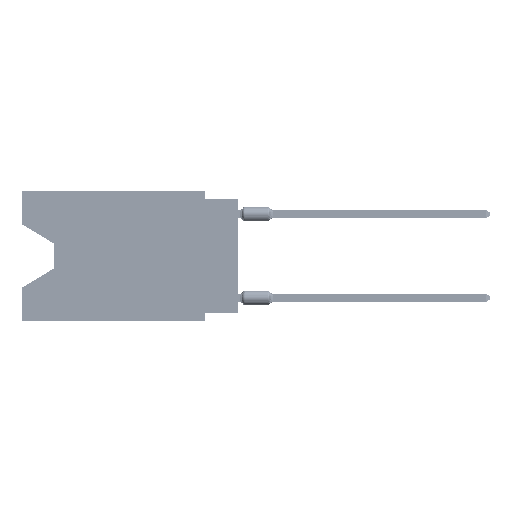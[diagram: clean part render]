
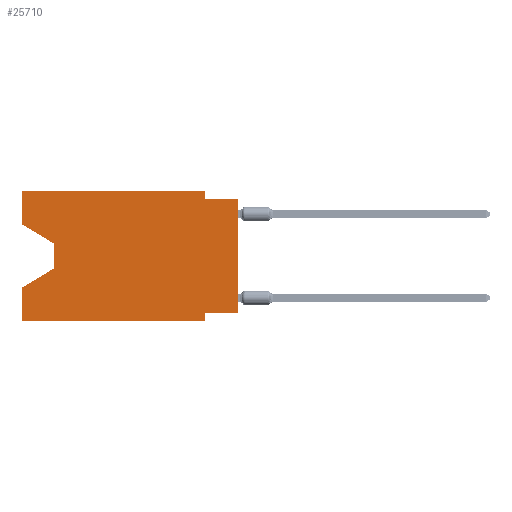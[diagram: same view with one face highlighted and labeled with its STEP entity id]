
A CAD part, left-side view. The second image highlights one B-rep face of the part: STEP entity #25710.
In plain terms, the highlighted planar face has unit normal (-1, 0, 0).
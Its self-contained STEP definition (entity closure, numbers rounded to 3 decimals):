
#931 = EDGE_CURVE ( 'NONE', #73443, #18157, #52153, .T. ) ;
#2565 = CARTESIAN_POINT ( 'NONE',  ( 0., 16.383, 0. ) ) ;
#4362 = DIRECTION ( 'NONE',  ( 0., 1., 0. ) ) ;
#6048 = PLANE ( 'NONE',  #30988 ) ;
#7263 = FACE_OUTER_BOUND ( 'NONE', #73727, .T. ) ;
#8220 = VERTEX_POINT ( 'NONE', #58531 ) ;
#8374 = VERTEX_POINT ( 'NONE', #29571 ) ;
#8647 = DIRECTION ( 'NONE',  ( 0., -1., 0. ) ) ;
#10878 = ORIENTED_EDGE ( 'NONE', *, *, #80492, .T. ) ;
#10929 = LINE ( 'NONE', #42342, #17483 ) ;
#10976 = DIRECTION ( 'NONE',  ( 0., 0., 1. ) ) ;
#11453 = DIRECTION ( 'NONE',  ( 0., 0., -1. ) ) ;
#12422 = DIRECTION ( 'NONE',  ( 0., -1., 0. ) ) ;
#15147 = ORIENTED_EDGE ( 'NONE', *, *, #59536, .F. ) ;
#16491 = CARTESIAN_POINT ( 'NONE',  ( 0., 13.97, -5.893 ) ) ;
#16906 = VERTEX_POINT ( 'NONE', #70762 ) ;
#17155 = LINE ( 'NONE', #54751, #63928 ) ;
#17483 = VECTOR ( 'NONE', #72112, 1000. ) ;
#18157 = VERTEX_POINT ( 'NONE', #69662 ) ;
#23806 = EDGE_CURVE ( 'NONE', #18157, #8220, #31807, .T. ) ;
#23817 = VERTEX_POINT ( 'NONE', #65637 ) ;
#23834 = CARTESIAN_POINT ( 'NONE',  ( 0., 13.97, -4.013 ) ) ;
#25710 = ADVANCED_FACE ( 'NONE', ( #7263 ), #6048, .F. ) ;
#25824 = ORIENTED_EDGE ( 'NONE', *, *, #931, .F. ) ;
#26356 = ORIENTED_EDGE ( 'NONE', *, *, #23806, .F. ) ;
#29123 = VECTOR ( 'NONE', #10976, 1000. ) ;
#29197 = ORIENTED_EDGE ( 'NONE', *, *, #75148, .F. ) ;
#29342 = EDGE_CURVE ( 'NONE', #74866, #76067, #44017, .T. ) ;
#29571 = CARTESIAN_POINT ( 'NONE',  ( 0., 13.97, -4.013 ) ) ;
#29937 = VERTEX_POINT ( 'NONE', #64129 ) ;
#29983 = DIRECTION ( 'NONE',  ( 0., 0., 1. ) ) ;
#30988 = AXIS2_PLACEMENT_3D ( 'NONE', #57633, #70462, #32436 ) ;
#31807 = LINE ( 'NONE', #50419, #73814 ) ;
#32436 = DIRECTION ( 'NONE',  ( 0., 0., -1. ) ) ;
#32648 = VECTOR ( 'NONE', #12422, 1000. ) ;
#33548 = VECTOR ( 'NONE', #8647, 1000. ) ;
#34141 = VECTOR ( 'NONE', #76958, 1000. ) ;
#34930 = CARTESIAN_POINT ( 'NONE',  ( 0., 16.383, 0. ) ) ;
#35953 = CARTESIAN_POINT ( 'NONE',  ( 0., 0., -9.271 ) ) ;
#35966 = CARTESIAN_POINT ( 'NONE',  ( 0., 2.54, -9.271 ) ) ;
#36505 = ORIENTED_EDGE ( 'NONE', *, *, #38215, .T. ) ;
#36901 = EDGE_CURVE ( 'NONE', #45316, #71982, #10929, .T. ) ;
#38215 = EDGE_CURVE ( 'NONE', #16906, #8374, #52815, .T. ) ;
#39100 = ORIENTED_EDGE ( 'NONE', *, *, #41524, .F. ) ;
#39624 = LINE ( 'NONE', #47450, #40632 ) ;
#40025 = DIRECTION ( 'NONE',  ( 0., 0., 1. ) ) ;
#40632 = VECTOR ( 'NONE', #40025, 1000. ) ;
#40779 = VECTOR ( 'NONE', #29983, 1000. ) ;
#41524 = EDGE_CURVE ( 'NONE', #76067, #29937, #17155, .T. ) ;
#42342 = CARTESIAN_POINT ( 'NONE',  ( 0., 13.97, -5.893 ) ) ;
#43422 = CARTESIAN_POINT ( 'NONE',  ( 0., 0., -0.635 ) ) ;
#44017 = LINE ( 'NONE', #79979, #76206 ) ;
#45316 = VERTEX_POINT ( 'NONE', #16491 ) ;
#47450 = CARTESIAN_POINT ( 'NONE',  ( 0., 0., 0. ) ) ;
#48983 = CARTESIAN_POINT ( 'NONE',  ( 0., 0., -0.635 ) ) ;
#50347 = EDGE_CURVE ( 'NONE', #16906, #73443, #80412, .T. ) ;
#50419 = CARTESIAN_POINT ( 'NONE',  ( 0., 2.54, 0. ) ) ;
#52153 = LINE ( 'NONE', #2565, #34141 ) ;
#52815 = LINE ( 'NONE', #54015, #63797 ) ;
#53298 = VERTEX_POINT ( 'NONE', #48983 ) ;
#53861 = EDGE_CURVE ( 'NONE', #23817, #29937, #71437, .T. ) ;
#54015 = CARTESIAN_POINT ( 'NONE',  ( 0., 16.383, -2.546 ) ) ;
#54292 = ORIENTED_EDGE ( 'NONE', *, *, #53861, .T. ) ;
#54751 = CARTESIAN_POINT ( 'NONE',  ( 0., 2.54, -9.906 ) ) ;
#55395 = LINE ( 'NONE', #43422, #32648 ) ;
#57633 = CARTESIAN_POINT ( 'NONE',  ( 0., 16.383, 0. ) ) ;
#57983 = ORIENTED_EDGE ( 'NONE', *, *, #36901, .T. ) ;
#58531 = CARTESIAN_POINT ( 'NONE',  ( 0., 2.54, -0.635 ) ) ;
#59536 = EDGE_CURVE ( 'NONE', #8220, #53298, #55395, .T. ) ;
#62073 = ORIENTED_EDGE ( 'NONE', *, *, #50347, .F. ) ;
#62603 = DIRECTION ( 'NONE',  ( 0., 0., -1. ) ) ;
#63797 = VECTOR ( 'NONE', #78829, 1000. ) ;
#63928 = VECTOR ( 'NONE', #62603, 1000. ) ;
#64083 = ORIENTED_EDGE ( 'NONE', *, *, #29342, .F. ) ;
#64129 = CARTESIAN_POINT ( 'NONE',  ( 0., 2.54, -9.906 ) ) ;
#64741 = CARTESIAN_POINT ( 'NONE',  ( 0., 16.383, 0. ) ) ;
#65151 = VECTOR ( 'NONE', #11453, 1000. ) ;
#65301 = LINE ( 'NONE', #23834, #65151 ) ;
#65637 = CARTESIAN_POINT ( 'NONE',  ( 0., 16.383, -9.906 ) ) ;
#65913 = ORIENTED_EDGE ( 'NONE', *, *, #71776, .T. ) ;
#67177 = LINE ( 'NONE', #34930, #29123 ) ;
#69662 = CARTESIAN_POINT ( 'NONE',  ( 0., 2.54, 0. ) ) ;
#70462 = DIRECTION ( 'NONE',  ( 1., 0., 0. ) ) ;
#70644 = CARTESIAN_POINT ( 'NONE',  ( 0., 16.383, -9.906 ) ) ;
#70762 = CARTESIAN_POINT ( 'NONE',  ( 0., 16.383, -2.546 ) ) ;
#71437 = LINE ( 'NONE', #70644, #33548 ) ;
#71776 = EDGE_CURVE ( 'NONE', #74866, #53298, #39624, .T. ) ;
#71982 = VERTEX_POINT ( 'NONE', #76724 ) ;
#72112 = DIRECTION ( 'NONE',  ( 0., 0.855, -0.519 ) ) ;
#73443 = VERTEX_POINT ( 'NONE', #64741 ) ;
#73727 = EDGE_LOOP ( 'NONE', ( #36505, #10878, #57983, #29197, #54292, #39100, #64083, #65913, #15147, #26356, #25824, #62073 ) ) ;
#73814 = VECTOR ( 'NONE', #75631, 1000. ) ;
#74630 = CARTESIAN_POINT ( 'NONE',  ( 0., 16.383, 0. ) ) ;
#74866 = VERTEX_POINT ( 'NONE', #35953 ) ;
#75148 = EDGE_CURVE ( 'NONE', #23817, #71982, #67177, .T. ) ;
#75631 = DIRECTION ( 'NONE',  ( 0., 0., -1. ) ) ;
#76067 = VERTEX_POINT ( 'NONE', #35966 ) ;
#76206 = VECTOR ( 'NONE', #4362, 1000. ) ;
#76724 = CARTESIAN_POINT ( 'NONE',  ( 0., 16.383, -7.36 ) ) ;
#76958 = DIRECTION ( 'NONE',  ( 0., -1., 0. ) ) ;
#78829 = DIRECTION ( 'NONE',  ( 0., -0.855, -0.519 ) ) ;
#79979 = CARTESIAN_POINT ( 'NONE',  ( 0., 0., -9.271 ) ) ;
#80412 = LINE ( 'NONE', #74630, #40779 ) ;
#80492 = EDGE_CURVE ( 'NONE', #8374, #45316, #65301, .T. ) ;
